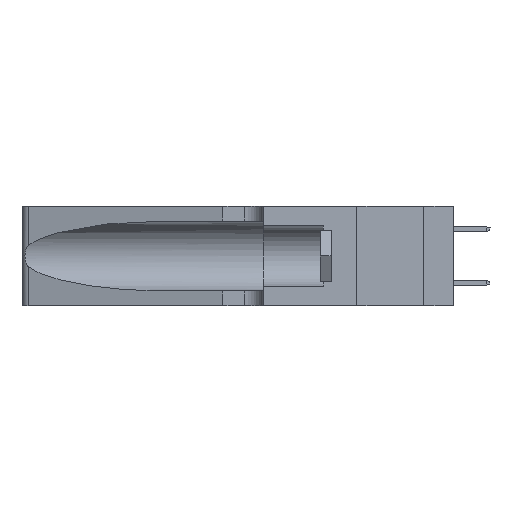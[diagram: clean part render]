
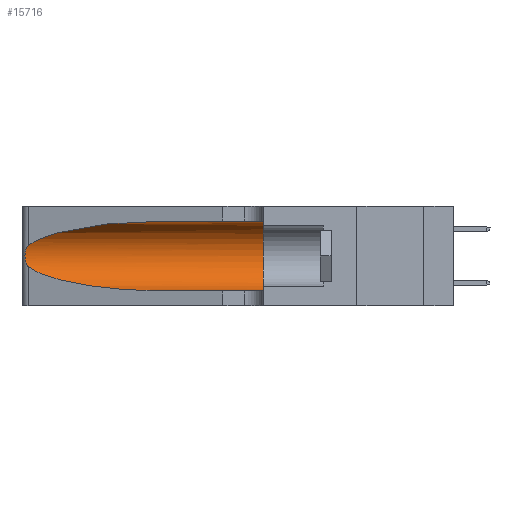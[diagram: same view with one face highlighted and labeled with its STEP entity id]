
A CAD part, left-side view. The second image highlights one B-rep face of the part: STEP entity #15716.
In plain terms, the highlighted cylindrical face has radius 3.308 mm (diameter 6.617 mm), a partial arc.
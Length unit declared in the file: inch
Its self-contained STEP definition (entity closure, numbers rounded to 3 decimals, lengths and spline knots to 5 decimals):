
#1 = CARTESIAN_POINT ( 'NONE',  ( 0.2373, 1.15595, 0.28018 ) ) ;
#358 = CARTESIAN_POINT ( 'NONE',  ( 0.25487, 1.22718, 0.14631 ) ) ;
#1047 = CARTESIAN_POINT ( 'NONE',  ( 0.1305, 0.72297, 0.31525 ) ) ;
#1540 = CARTESIAN_POINT ( 'NONE',  ( 0.26018, 1.23835, 0.19895 ) ) ;
#1757 = VERTEX_POINT ( 'NONE', #14090 ) ;
#2053 = EDGE_CURVE ( 'NONE', #14408, #14355, #16667, .T. ) ;
#2349 = AXIS2_PLACEMENT_3D ( 'NONE', #13641, #6388, #15253 ) ;
#3185 = CARTESIAN_POINT ( 'NONE',  ( 0.1305, 1.61858, 0.05475 ) ) ;
#3539 = ORIENTED_EDGE ( 'NONE', *, *, #4037, .F. ) ;
#4037 = EDGE_CURVE ( 'NONE', #4807, #7595, #7841, .T. ) ;
#4222 = EDGE_CURVE ( 'NONE', #13408, #14408, #15852, .T. ) ;
#4476 = CARTESIAN_POINT ( 'NONE',  ( 0.25789, 1.23486, 0.15765 ) ) ;
#4578 = CARTESIAN_POINT ( 'NONE',  ( 0.25787, 1.23484, 0.2124 ) ) ;
#4807 = VERTEX_POINT ( 'NONE', #1047 ) ;
#5267 = ORIENTED_EDGE ( 'NONE', *, *, #18389, .T. ) ;
#6288 = DIRECTION ( 'NONE',  ( 0., -1., 0. ) ) ;
#6388 = DIRECTION ( 'NONE',  ( 0., 1., 0. ) ) ;
#6544 = CARTESIAN_POINT ( 'NONE',  ( 0.25487, 1.22718, 0.14631 ) ) ;
#6733 = CARTESIAN_POINT ( 'NONE',  ( 0.2373, 1.15595, 0.08982 ) ) ;
#6822 = CARTESIAN_POINT ( 'NONE',  ( 0.18966, 0.96281, 0.05475 ) ) ;
#7068 = CARTESIAN_POINT ( 'NONE',  ( 0.25487, 1.22718, 0.14631 ) ) ;
#7541 = DIRECTION ( 'NONE',  ( 0., -1., 0. ) ) ;
#7595 = VERTEX_POINT ( 'NONE', #19742 ) ;
#7817 = ORIENTED_EDGE ( 'NONE', *, *, #4222, .T. ) ;
#7841 = LINE ( 'NONE', #19680, #12795 ) ;
#7976 = CARTESIAN_POINT ( 'NONE',  ( 0.25854, 1.2359, 0.20912 ) ) ;
#9221 = VECTOR ( 'NONE', #6288, 39.37008 ) ;
#9734 = DIRECTION ( 'NONE',  ( 0., -1., 0. ) ) ;
#9866 = CARTESIAN_POINT ( 'NONE',  ( 0.1305, 0.35, 0.05475 ) ) ;
#10020 = DIRECTION ( 'NONE',  ( 0., 0., -1. ) ) ;
#10554 = EDGE_CURVE ( 'NONE', #7595, #14355, #14456, .T. ) ;
#11014 = B_SPLINE_CURVE_WITH_KNOTS ( 'NONE', 3,
 ( #13625, #18236, #16752, #4578, #7976, #1540, #14022, #18429, #15340, #15241, #4476, #13822, #12235, #358 ),
 .UNSPECIFIED., .F., .F.,
 ( 4, 2, 2, 2, 2, 2, 4 ),
 ( 0., 0.00027, 0.00053, 0.00107, 0.0016, 0.00187, 0.00214 ),
 .UNSPECIFIED. ) ;
#11018 = CARTESIAN_POINT ( 'NONE',  ( 0.1305, 0.72297, 0.31525 ) ) ;
#12039 = EDGE_CURVE ( 'NONE', #1757, #13408, #11014, .T. ) ;
#12148 = ORIENTED_EDGE ( 'NONE', *, *, #12039, .T. ) ;
#12235 = CARTESIAN_POINT ( 'NONE',  ( 0.25555, 1.22993, 0.14849 ) ) ;
#12472 = EDGE_LOOP ( 'NONE', ( #5267, #12148, #7817, #14732, #18153, #3539 ) ) ;
#12795 = VECTOR ( 'NONE', #7541, 39.37008 ) ;
#13408 = VERTEX_POINT ( 'NONE', #7068 ) ;
#13625 = CARTESIAN_POINT ( 'NONE',  ( 0.25487, 1.22718, 0.22369 ) ) ;
#13641 = CARTESIAN_POINT ( 'NONE',  ( 0.1305, 0.35, 0.185 ) ) ;
#13822 = CARTESIAN_POINT ( 'NONE',  ( 0.25639, 1.23186, 0.15144 ) ) ;
#14022 = CARTESIAN_POINT ( 'NONE',  ( 0.26075, 1.23896, 0.19203 ) ) ;
#14090 = CARTESIAN_POINT ( 'NONE',  ( 0.25487, 1.22718, 0.22369 ) ) ;
#14355 = VERTEX_POINT ( 'NONE', #9866 ) ;
#14408 = VERTEX_POINT ( 'NONE', #16314 ) ;
#14456 = CIRCLE ( 'NONE', #2349, 0.13025 ) ;
#14732 = ORIENTED_EDGE ( 'NONE', *, *, #2053, .T. ) ;
#15241 = CARTESIAN_POINT ( 'NONE',  ( 0.25856, 1.23593, 0.16098 ) ) ;
#15253 = DIRECTION ( 'NONE',  ( 0., 0., 1. ) ) ;
#15340 = CARTESIAN_POINT ( 'NONE',  ( 0.26017, 1.23833, 0.17102 ) ) ;
#15508 =( BOUNDED_CURVE ( )  B_SPLINE_CURVE ( 3, ( #11018, #18197, #1, #15605 ),
 .UNSPECIFIED., .F., .F. ) 
 B_SPLINE_CURVE_WITH_KNOTS ( ( 4, 4 ),
 ( 1.5708, 2.84003 ),
 .UNSPECIFIED. ) 
 CURVE ( )  GEOMETRIC_REPRESENTATION_ITEM ( )  RATIONAL_B_SPLINE_CURVE ( ( 1., 0.87, 0.87, 1. ) ) 
 REPRESENTATION_ITEM ( '' )  );
#15516 = CARTESIAN_POINT ( 'NONE',  ( 0.1305, 0.72297, 0.05475 ) ) ;
#15605 = CARTESIAN_POINT ( 'NONE',  ( 0.25487, 1.22718, 0.22369 ) ) ;
#15716 = ADVANCED_FACE ( 'NONE', ( #16011 ), #17329, .F. ) ;
#15732 = CARTESIAN_POINT ( 'NONE',  ( 0.1305, 1.61858, 0.185 ) ) ;
#15852 =( BOUNDED_CURVE ( )  B_SPLINE_CURVE ( 3, ( #6544, #6733, #6822, #15516 ),
 .UNSPECIFIED., .F., .F. ) 
 B_SPLINE_CURVE_WITH_KNOTS ( ( 4, 4 ),
 ( 3.44316, 4.71239 ),
 .UNSPECIFIED. ) 
 CURVE ( )  GEOMETRIC_REPRESENTATION_ITEM ( )  RATIONAL_B_SPLINE_CURVE ( ( 1., 0.87, 0.87, 1. ) ) 
 REPRESENTATION_ITEM ( '' )  );
#16011 = FACE_OUTER_BOUND ( 'NONE', #12472, .T. ) ;
#16314 = CARTESIAN_POINT ( 'NONE',  ( 0.1305, 0.72297, 0.05475 ) ) ;
#16667 = LINE ( 'NONE', #3185, #9221 ) ;
#16752 = CARTESIAN_POINT ( 'NONE',  ( 0.25639, 1.23184, 0.21858 ) ) ;
#17329 = CYLINDRICAL_SURFACE ( 'NONE', #17485, 0.13025 ) ;
#17485 = AXIS2_PLACEMENT_3D ( 'NONE', #15732, #9734, #10020 ) ;
#18153 = ORIENTED_EDGE ( 'NONE', *, *, #10554, .F. ) ;
#18197 = CARTESIAN_POINT ( 'NONE',  ( 0.18966, 0.96281, 0.31525 ) ) ;
#18236 = CARTESIAN_POINT ( 'NONE',  ( 0.25555, 1.22994, 0.2215 ) ) ;
#18389 = EDGE_CURVE ( 'NONE', #4807, #1757, #15508, .T. ) ;
#18429 = CARTESIAN_POINT ( 'NONE',  ( 0.26075, 1.23896, 0.178 ) ) ;
#19680 = CARTESIAN_POINT ( 'NONE',  ( 0.1305, 1.61858, 0.31525 ) ) ;
#19742 = CARTESIAN_POINT ( 'NONE',  ( 0.1305, 0.35, 0.31525 ) ) ;
